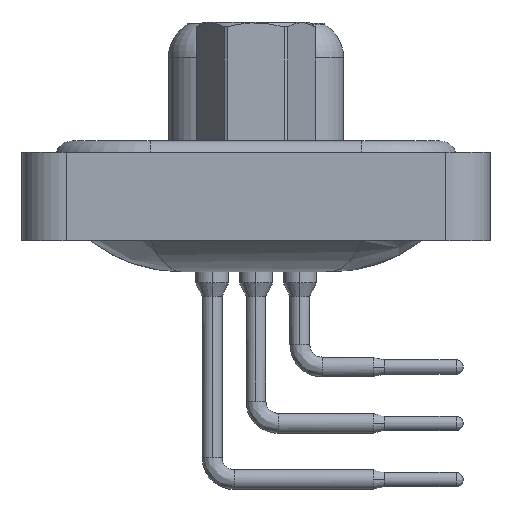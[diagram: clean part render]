
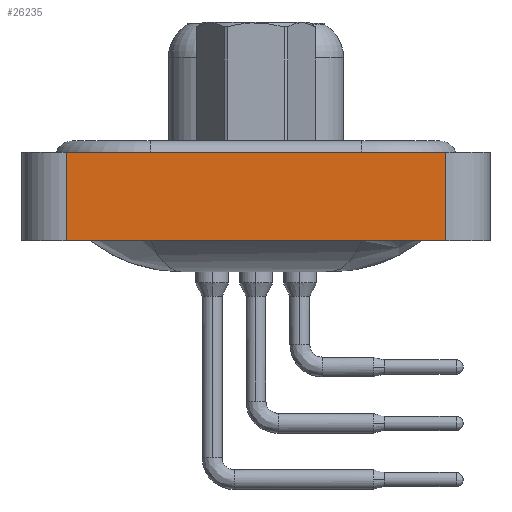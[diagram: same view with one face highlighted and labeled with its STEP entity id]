
A CAD part, left-side view. The second image highlights one B-rep face of the part: STEP entity #26235.
In plain terms, the highlighted planar face has unit normal (-1, 0, 0).
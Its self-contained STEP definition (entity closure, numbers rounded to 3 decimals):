
#745 = VECTOR ( 'NONE', #13163, 1000. ) ;
#1205 = CARTESIAN_POINT ( 'NONE',  ( -7.285, -8.55, 0.4 ) ) ;
#2249 = LINE ( 'NONE', #22730, #745 ) ;
#4696 = CARTESIAN_POINT ( 'NONE',  ( -7.285, -8.55, -3.6 ) ) ;
#5196 = EDGE_CURVE ( 'NONE', #30699, #14393, #5925, .T. ) ;
#5925 = LINE ( 'NONE', #11018, #12298 ) ;
#6791 = FACE_OUTER_BOUND ( 'NONE', #19764, .T. ) ;
#7269 = VECTOR ( 'NONE', #20461, 1000. ) ;
#7501 = DIRECTION ( 'NONE',  ( 0., 0., 1. ) ) ;
#9548 = DIRECTION ( 'NONE',  ( 0., 0., 1. ) ) ;
#10571 = EDGE_CURVE ( 'NONE', #14393, #10778, #23895, .T. ) ;
#10778 = VERTEX_POINT ( 'NONE', #15212 ) ;
#11018 = CARTESIAN_POINT ( 'NONE',  ( -7.285, -8.55, -3.6 ) ) ;
#11788 = EDGE_CURVE ( 'NONE', #27043, #10778, #27196, .T. ) ;
#12298 = VECTOR ( 'NONE', #18033, 1000. ) ;
#12352 = AXIS2_PLACEMENT_3D ( 'NONE', #26596, #21881, #7501 ) ;
#13135 = ORIENTED_EDGE ( 'NONE', *, *, #5196, .T. ) ;
#13163 = DIRECTION ( 'NONE',  ( 0., 0., 1. ) ) ;
#13987 = CARTESIAN_POINT ( 'NONE',  ( -7.285, 8.55, -3.6 ) ) ;
#14393 = VERTEX_POINT ( 'NONE', #23616 ) ;
#14814 = ORIENTED_EDGE ( 'NONE', *, *, #26507, .F. ) ;
#15212 = CARTESIAN_POINT ( 'NONE',  ( -7.285, -8.55, 0.4 ) ) ;
#17013 = PLANE ( 'NONE',  #12352 ) ;
#17461 = VECTOR ( 'NONE', #9548, 1000. ) ;
#18033 = DIRECTION ( 'NONE',  ( 0., -1., 0. ) ) ;
#19043 = ORIENTED_EDGE ( 'NONE', *, *, #10571, .T. ) ;
#19764 = EDGE_LOOP ( 'NONE', ( #19043, #21138, #14814, #13135 ) ) ;
#20461 = DIRECTION ( 'NONE',  ( 0., -1., 0. ) ) ;
#21138 = ORIENTED_EDGE ( 'NONE', *, *, #11788, .F. ) ;
#21205 = CARTESIAN_POINT ( 'NONE',  ( -7.285, 8.55, 0.4 ) ) ;
#21881 = DIRECTION ( 'NONE',  ( -1., 0., 0. ) ) ;
#22730 = CARTESIAN_POINT ( 'NONE',  ( -7.285, 8.55, -3.6 ) ) ;
#23616 = CARTESIAN_POINT ( 'NONE',  ( -7.285, -8.55, -3.6 ) ) ;
#23895 = LINE ( 'NONE', #4696, #17461 ) ;
#26235 = ADVANCED_FACE ( 'NONE', ( #6791 ), #17013, .T. ) ;
#26507 = EDGE_CURVE ( 'NONE', #30699, #27043, #2249, .T. ) ;
#26596 = CARTESIAN_POINT ( 'NONE',  ( -7.285, -8.55, -3.6 ) ) ;
#27043 = VERTEX_POINT ( 'NONE', #21205 ) ;
#27196 = LINE ( 'NONE', #1205, #7269 ) ;
#30699 = VERTEX_POINT ( 'NONE', #13987 ) ;
